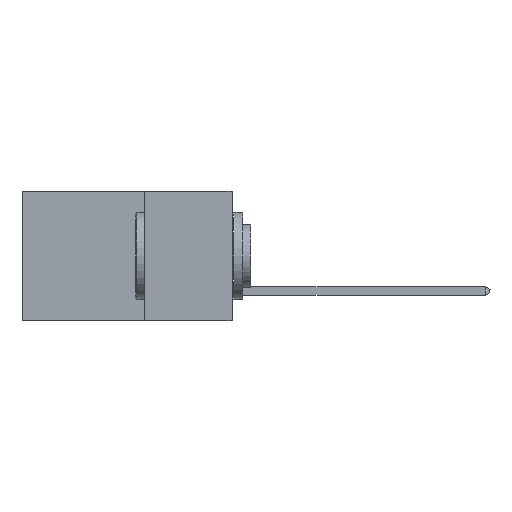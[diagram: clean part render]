
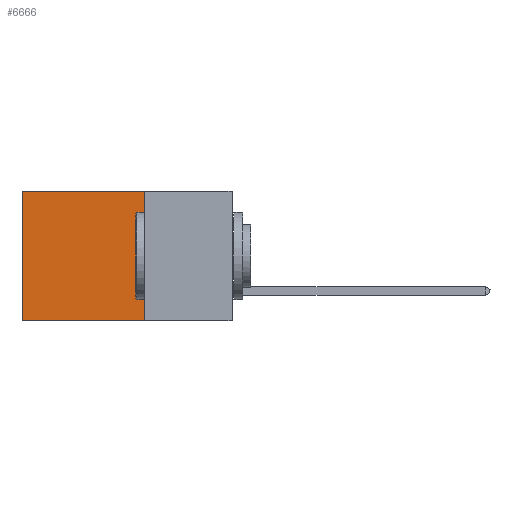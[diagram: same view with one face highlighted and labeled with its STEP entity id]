
A CAD part, left-side view. The second image highlights one B-rep face of the part: STEP entity #6666.
In plain terms, the highlighted planar face has unit normal (-1, 0, 0).
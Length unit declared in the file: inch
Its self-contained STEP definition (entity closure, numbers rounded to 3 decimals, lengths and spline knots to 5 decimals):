
#1570 = CARTESIAN_POINT ( 'NONE',  ( 0.2875, 0.25, 0. ) ) ;
#3508 = EDGE_CURVE ( 'NONE', #10310, #28966, #4950, .T. ) ;
#4076 = VERTEX_POINT ( 'NONE', #31175 ) ;
#4418 = EDGE_CURVE ( 'NONE', #4076, #10310, #5896, .T. ) ;
#4867 = VECTOR ( 'NONE', #15658, 39.37008 ) ;
#4950 = LINE ( 'NONE', #17680, #29453 ) ;
#4956 = DIRECTION ( 'NONE',  ( 0., 0., -1. ) ) ;
#5896 = LINE ( 'NONE', #25587, #4867 ) ;
#6399 = ORIENTED_EDGE ( 'NONE', *, *, #3508, .T. ) ;
#6666 = ADVANCED_FACE ( 'NONE', ( #38297 ), #7878, .F. ) ;
#7878 = PLANE ( 'NONE',  #26476 ) ;
#8525 = ORIENTED_EDGE ( 'NONE', *, *, #8628, .F. ) ;
#8628 = EDGE_CURVE ( 'NONE', #4076, #33990, #24651, .T. ) ;
#10310 = VERTEX_POINT ( 'NONE', #28753 ) ;
#12247 = VECTOR ( 'NONE', #14550, 39.37008 ) ;
#14550 = DIRECTION ( 'NONE',  ( 0., 1., 0. ) ) ;
#15658 = DIRECTION ( 'NONE',  ( 0., 1., 0. ) ) ;
#17171 = DIRECTION ( 'NONE',  ( 1., 0., 0. ) ) ;
#17680 = CARTESIAN_POINT ( 'NONE',  ( 0.2875, 0.6, 0. ) ) ;
#21354 = DIRECTION ( 'NONE',  ( 0., 0., -1. ) ) ;
#23140 = ORIENTED_EDGE ( 'NONE', *, *, #26866, .F. ) ;
#24278 = LINE ( 'NONE', #29335, #12247 ) ;
#24424 = CARTESIAN_POINT ( 'NONE',  ( 0.2875, 0.6, -0.37 ) ) ;
#24651 = LINE ( 'NONE', #1570, #25642 ) ;
#25587 = CARTESIAN_POINT ( 'NONE',  ( 0.2875, 0.25, 0. ) ) ;
#25642 = VECTOR ( 'NONE', #4956, 39.37008 ) ;
#26476 = AXIS2_PLACEMENT_3D ( 'NONE', #27183, #17171, #21354 ) ;
#26866 = EDGE_CURVE ( 'NONE', #33990, #28966, #24278, .T. ) ;
#27183 = CARTESIAN_POINT ( 'NONE',  ( 0.2875, 0.25, 0. ) ) ;
#28753 = CARTESIAN_POINT ( 'NONE',  ( 0.2875, 0.6, 0. ) ) ;
#28966 = VERTEX_POINT ( 'NONE', #24424 ) ;
#29335 = CARTESIAN_POINT ( 'NONE',  ( 0.2875, 0.25, -0.37 ) ) ;
#29453 = VECTOR ( 'NONE', #30447, 39.37008 ) ;
#30447 = DIRECTION ( 'NONE',  ( 0., 0., -1. ) ) ;
#31175 = CARTESIAN_POINT ( 'NONE',  ( 0.2875, 0.25, 0. ) ) ;
#33990 = VERTEX_POINT ( 'NONE', #38551 ) ;
#35856 = ORIENTED_EDGE ( 'NONE', *, *, #4418, .T. ) ;
#37339 = EDGE_LOOP ( 'NONE', ( #6399, #23140, #8525, #35856 ) ) ;
#38297 = FACE_OUTER_BOUND ( 'NONE', #37339, .T. ) ;
#38551 = CARTESIAN_POINT ( 'NONE',  ( 0.2875, 0.25, -0.37 ) ) ;
